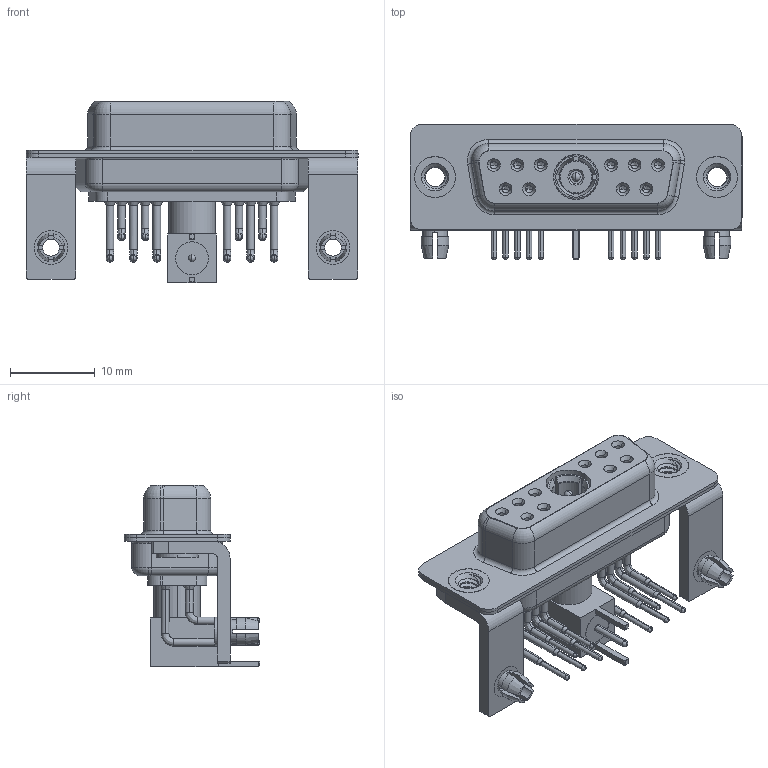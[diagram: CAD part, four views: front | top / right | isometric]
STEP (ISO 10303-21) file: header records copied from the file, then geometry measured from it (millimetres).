
FILE_DESCRIPTION (( 'STEP AP203' ), '1' );
FILE_NAME ('630-11W1240-7N3.STEP', '2022-05-31T09:59:39', ( '' ), ( '' ), 'SwSTEP 2.0', 'SolidWorks 2020', '' );
FILE_SCHEMA (( 'CONFIG_CONTROL_DESIGN' ));
Length unit declared in the file: millimetre
Products named in the file (16): 630Combo Contact Row 2; 630Combo Housing_11W1; 630Combo Stabilizer Bracket; RA Back Shell; 630Combo Shell Rear_15 Contacts; 630Combo Board Lock; Insulator RA Pin; Locking Collar; 630-11W1240-7N3; Co-Ax Plug_RA PC Tail; Pin_RA; 630Combo Threaded Rivet_3; Co-Ax Plug Assy_RA; 630Combo Contact Row 1; Insulator Pin_Straight PC Tail; 630Combo Shell Front_15 Contacts
Assembly tree (26 placements, depth 3):
  630-11W1240-7N3
    630Combo Housing_11W1
    630Combo Shell Front_15 Contacts
    630Combo Shell Rear_15 Contacts
    630Combo Threaded Rivet_3  x2
    630Combo Stabilizer Bracket  x2
    630Combo Board Lock  x2
    Co-Ax Plug Assy_RA
      Co-Ax Plug_RA PC Tail
      Insulator Pin_Straight PC Tail
      Pin_RA
      Locking Collar
      RA Back Shell
      Insulator RA Pin
    630Combo Contact Row 1  x6
    630Combo Contact Row 2  x4
Bounding box: 39.2 x 16 x 21.41 mm (x, y, z)
Volume: 3115.6 mm3; surface area: 7690.6 mm2
Topology: 25 solids, 25 shells, 1109 faces, 2786 edges, 1758 vertices
Faces by surface type: cylinder 482, plane 352, cone 161, torus 63, bspline 47, sphere 4
Entity records: 24125 total; most frequent: CARTESIAN_POINT 5474, DIRECTION 3768, ORIENTED_EDGE 3308, EDGE_CURVE 1654, AXIS2_PLACEMENT_3D 1527, VERTEX_POINT 1053, CIRCLE 819, EDGE_LOOP 801
